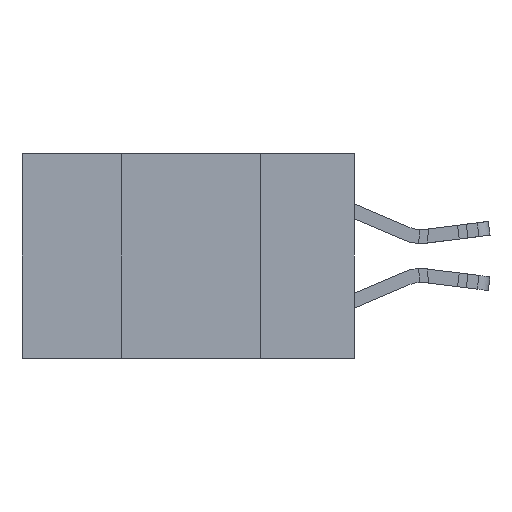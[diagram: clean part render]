
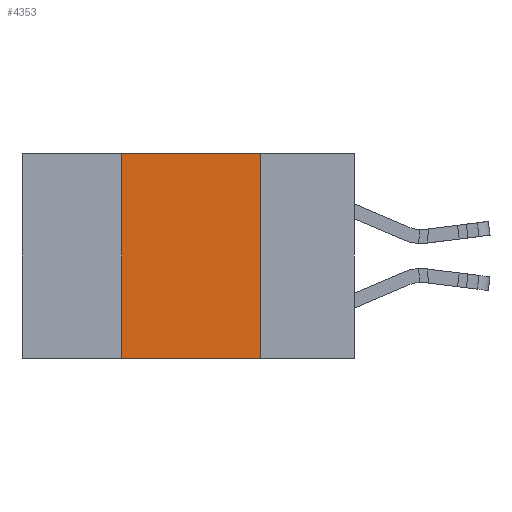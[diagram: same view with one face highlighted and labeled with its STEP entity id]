
A CAD part, left-side view. The second image highlights one B-rep face of the part: STEP entity #4353.
In plain terms, the highlighted planar face has unit normal (-1, 0, 0).
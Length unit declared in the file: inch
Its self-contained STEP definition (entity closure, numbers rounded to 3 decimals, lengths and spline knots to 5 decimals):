
#67 = ORIENTED_EDGE ( 'NONE', *, *, #25006, .F. ) ;
#211 = DIRECTION ( 'NONE',  ( 1., 0., 0. ) ) ;
#597 = DIRECTION ( 'NONE',  ( 0., 0., -1. ) ) ;
#991 = EDGE_CURVE ( 'NONE', #15547, #25130, #4067, .T. ) ;
#1287 = LINE ( 'NONE', #24337, #18930 ) ;
#1464 = LINE ( 'NONE', #9671, #13675 ) ;
#2746 = CARTESIAN_POINT ( 'NONE',  ( 0., 0.6, 0. ) ) ;
#2815 = VERTEX_POINT ( 'NONE', #10425 ) ;
#4067 = LINE ( 'NONE', #15751, #6677 ) ;
#4353 = ADVANCED_FACE ( 'NONE', ( #25032 ), #12697, .F. ) ;
#5816 = DIRECTION ( 'NONE',  ( 0., -1., 0. ) ) ;
#6677 = VECTOR ( 'NONE', #5816, 39.37008 ) ;
#6771 = EDGE_CURVE ( 'NONE', #2815, #25130, #9063, .T. ) ;
#6854 = EDGE_LOOP ( 'NONE', ( #11592, #67, #11421, #14336 ) ) ;
#7870 = CARTESIAN_POINT ( 'NONE',  ( 0., 0.42, 0. ) ) ;
#9063 = LINE ( 'NONE', #14827, #21254 ) ;
#9354 = DIRECTION ( 'NONE',  ( 0., -1., 0. ) ) ;
#9671 = CARTESIAN_POINT ( 'NONE',  ( 0., 0.42, -0.37 ) ) ;
#10425 = CARTESIAN_POINT ( 'NONE',  ( 0., 0.17, 0. ) ) ;
#11421 = ORIENTED_EDGE ( 'NONE', *, *, #21074, .F. ) ;
#11592 = ORIENTED_EDGE ( 'NONE', *, *, #6771, .F. ) ;
#12697 = PLANE ( 'NONE',  #24168 ) ;
#13675 = VECTOR ( 'NONE', #17823, 39.37008 ) ;
#14336 = ORIENTED_EDGE ( 'NONE', *, *, #991, .T. ) ;
#14827 = CARTESIAN_POINT ( 'NONE',  ( 0., 0.17, -0.37 ) ) ;
#15547 = VERTEX_POINT ( 'NONE', #21746 ) ;
#15751 = CARTESIAN_POINT ( 'NONE',  ( 0., 0.6, -0.37 ) ) ;
#16647 = VERTEX_POINT ( 'NONE', #7870 ) ;
#17093 = DIRECTION ( 'NONE',  ( 0., 0., -1. ) ) ;
#17823 = DIRECTION ( 'NONE',  ( 0., 0., 1. ) ) ;
#18930 = VECTOR ( 'NONE', #9354, 39.37008 ) ;
#21074 = EDGE_CURVE ( 'NONE', #15547, #16647, #1464, .T. ) ;
#21254 = VECTOR ( 'NONE', #17093, 39.37008 ) ;
#21746 = CARTESIAN_POINT ( 'NONE',  ( 0., 0.42, -0.37 ) ) ;
#24168 = AXIS2_PLACEMENT_3D ( 'NONE', #2746, #211, #597 ) ;
#24337 = CARTESIAN_POINT ( 'NONE',  ( 0., 0.6, 0. ) ) ;
#24469 = CARTESIAN_POINT ( 'NONE',  ( 0., 0.17, -0.37 ) ) ;
#25006 = EDGE_CURVE ( 'NONE', #16647, #2815, #1287, .T. ) ;
#25032 = FACE_OUTER_BOUND ( 'NONE', #6854, .T. ) ;
#25130 = VERTEX_POINT ( 'NONE', #24469 ) ;
